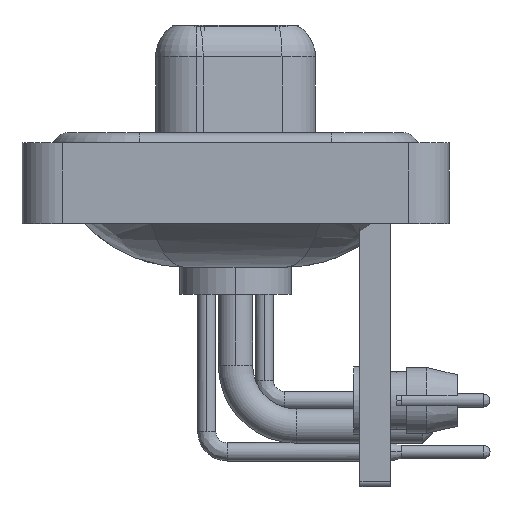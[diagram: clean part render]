
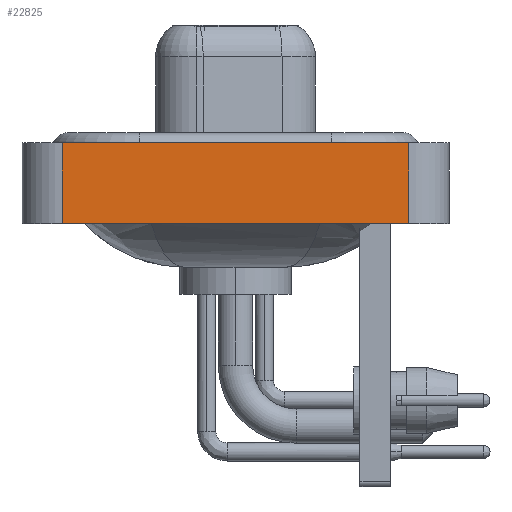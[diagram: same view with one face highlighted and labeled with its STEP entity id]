
A CAD part, left-side view. The second image highlights one B-rep face of the part: STEP entity #22825.
In plain terms, the highlighted planar face has unit normal (-1, 0, 0).
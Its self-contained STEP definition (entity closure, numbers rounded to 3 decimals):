
#240 = DIRECTION ( 'NONE',  ( 0., -1., 0. ) ) ;
#1108 = EDGE_CURVE ( 'NONE', #6342, #12394, #12501, .T. ) ;
#1325 = ORIENTED_EDGE ( 'NONE', *, *, #7876, .T. ) ;
#2096 = CARTESIAN_POINT ( 'NONE',  ( -7.35, -8.55, -3.6 ) ) ;
#2704 = LINE ( 'NONE', #10364, #3477 ) ;
#2843 = DIRECTION ( 'NONE',  ( 0., 0., 1. ) ) ;
#3477 = VECTOR ( 'NONE', #2843, 1000. ) ;
#4202 = CARTESIAN_POINT ( 'NONE',  ( -7.35, 8.55, -3.6 ) ) ;
#5652 = VECTOR ( 'NONE', #240, 1000. ) ;
#5902 = DIRECTION ( 'NONE',  ( 0., 0., 1. ) ) ;
#5934 = VERTEX_POINT ( 'NONE', #12905 ) ;
#6160 = CARTESIAN_POINT ( 'NONE',  ( -7.35, -8.55, -3.6 ) ) ;
#6342 = VERTEX_POINT ( 'NONE', #4202 ) ;
#7185 = ORIENTED_EDGE ( 'NONE', *, *, #9390, .F. ) ;
#7674 = AXIS2_PLACEMENT_3D ( 'NONE', #6160, #21761, #5902 ) ;
#7876 = EDGE_CURVE ( 'NONE', #12394, #12500, #2704, .T. ) ;
#8212 = CARTESIAN_POINT ( 'NONE',  ( -7.35, -8.55, 0.4 ) ) ;
#9390 = EDGE_CURVE ( 'NONE', #6342, #5934, #10877, .T. ) ;
#10046 = CARTESIAN_POINT ( 'NONE',  ( -7.35, -8.55, 0.4 ) ) ;
#10364 = CARTESIAN_POINT ( 'NONE',  ( -7.35, -8.55, -3.6 ) ) ;
#10877 = LINE ( 'NONE', #20983, #22722 ) ;
#12394 = VERTEX_POINT ( 'NONE', #2096 ) ;
#12500 = VERTEX_POINT ( 'NONE', #8212 ) ;
#12501 = LINE ( 'NONE', #14316, #5652 ) ;
#12905 = CARTESIAN_POINT ( 'NONE',  ( -7.35, 8.55, 0.4 ) ) ;
#14233 = FACE_OUTER_BOUND ( 'NONE', #14435, .T. ) ;
#14316 = CARTESIAN_POINT ( 'NONE',  ( -7.35, -8.55, -3.6 ) ) ;
#14435 = EDGE_LOOP ( 'NONE', ( #1325, #15102, #7185, #17726 ) ) ;
#15102 = ORIENTED_EDGE ( 'NONE', *, *, #15139, .F. ) ;
#15139 = EDGE_CURVE ( 'NONE', #5934, #12500, #22314, .T. ) ;
#17726 = ORIENTED_EDGE ( 'NONE', *, *, #1108, .T. ) ;
#18564 = DIRECTION ( 'NONE',  ( 0., 0., 1. ) ) ;
#20983 = CARTESIAN_POINT ( 'NONE',  ( -7.35, 8.55, -3.6 ) ) ;
#21761 = DIRECTION ( 'NONE',  ( -1., 0., 0. ) ) ;
#22314 = LINE ( 'NONE', #10046, #24993 ) ;
#22722 = VECTOR ( 'NONE', #18564, 1000. ) ;
#22825 = ADVANCED_FACE ( 'NONE', ( #14233 ), #23667, .T. ) ;
#23667 = PLANE ( 'NONE',  #7674 ) ;
#23970 = DIRECTION ( 'NONE',  ( 0., -1., 0. ) ) ;
#24993 = VECTOR ( 'NONE', #23970, 1000. ) ;
